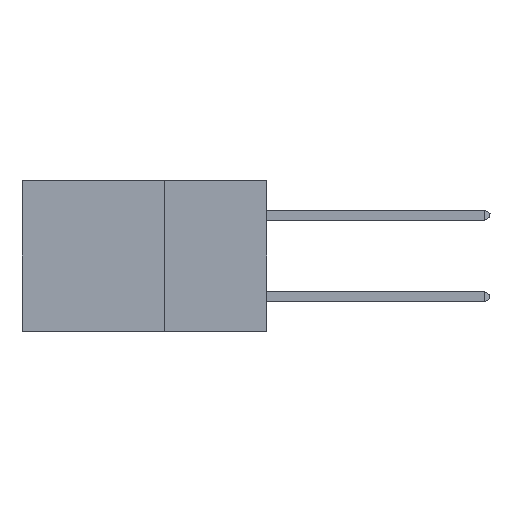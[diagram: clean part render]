
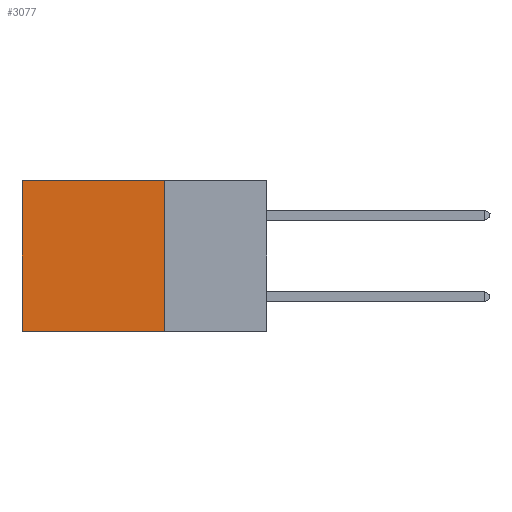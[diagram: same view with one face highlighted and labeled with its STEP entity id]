
A CAD part, left-side view. The second image highlights one B-rep face of the part: STEP entity #3077.
In plain terms, the highlighted planar face has unit normal (-1, 0, 0).
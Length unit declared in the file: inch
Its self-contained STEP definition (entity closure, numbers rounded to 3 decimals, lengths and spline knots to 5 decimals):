
#254 = CARTESIAN_POINT ( 'NONE',  ( 0.2875, 0.25, 0. ) ) ;
#445 = CARTESIAN_POINT ( 'NONE',  ( 0.2875, 0.6, 0. ) ) ;
#1049 = ORIENTED_EDGE ( 'NONE', *, *, #9684, .T. ) ;
#1185 = EDGE_CURVE ( 'NONE', #12153, #7019, #10264, .T. ) ;
#1751 = DIRECTION ( 'NONE',  ( 0., 0., -1. ) ) ;
#2098 = VECTOR ( 'NONE', #1751, 39.37008 ) ;
#2467 = LINE ( 'NONE', #7668, #2098 ) ;
#2470 = CARTESIAN_POINT ( 'NONE',  ( 0.2875, 0.25, -0.37 ) ) ;
#2887 = DIRECTION ( 'NONE',  ( 0., 1., 0. ) ) ;
#2899 = FACE_OUTER_BOUND ( 'NONE', #4478, .T. ) ;
#2956 = CARTESIAN_POINT ( 'NONE',  ( 0.2875, 0.25, 0. ) ) ;
#3077 = ADVANCED_FACE ( 'NONE', ( #2899 ), #14508, .F. ) ;
#3376 = ORIENTED_EDGE ( 'NONE', *, *, #3993, .T. ) ;
#3567 = VERTEX_POINT ( 'NONE', #8154 ) ;
#3993 = EDGE_CURVE ( 'NONE', #12153, #4284, #11089, .T. ) ;
#4284 = VERTEX_POINT ( 'NONE', #445 ) ;
#4478 = EDGE_LOOP ( 'NONE', ( #1049, #7407, #13186, #3376 ) ) ;
#4603 = VECTOR ( 'NONE', #8469, 39.37008 ) ;
#5119 = VECTOR ( 'NONE', #2887, 39.37008 ) ;
#6081 = DIRECTION ( 'NONE',  ( 0., 1., 0. ) ) ;
#7019 = VERTEX_POINT ( 'NONE', #8833 ) ;
#7407 = ORIENTED_EDGE ( 'NONE', *, *, #12311, .F. ) ;
#7668 = CARTESIAN_POINT ( 'NONE',  ( 0.2875, 0.6, 0. ) ) ;
#8104 = LINE ( 'NONE', #2470, #10340 ) ;
#8154 = CARTESIAN_POINT ( 'NONE',  ( 0.2875, 0.6, -0.37 ) ) ;
#8469 = DIRECTION ( 'NONE',  ( 0., 0., -1. ) ) ;
#8833 = CARTESIAN_POINT ( 'NONE',  ( 0.2875, 0.25, -0.37 ) ) ;
#9684 = EDGE_CURVE ( 'NONE', #4284, #3567, #2467, .T. ) ;
#10264 = LINE ( 'NONE', #254, #4603 ) ;
#10340 = VECTOR ( 'NONE', #6081, 39.37008 ) ;
#11084 = AXIS2_PLACEMENT_3D ( 'NONE', #14716, #14483, #14467 ) ;
#11089 = LINE ( 'NONE', #2956, #5119 ) ;
#12153 = VERTEX_POINT ( 'NONE', #12570 ) ;
#12311 = EDGE_CURVE ( 'NONE', #7019, #3567, #8104, .T. ) ;
#12570 = CARTESIAN_POINT ( 'NONE',  ( 0.2875, 0.25, 0. ) ) ;
#13186 = ORIENTED_EDGE ( 'NONE', *, *, #1185, .F. ) ;
#14467 = DIRECTION ( 'NONE',  ( 0., 0., -1. ) ) ;
#14483 = DIRECTION ( 'NONE',  ( 1., 0., 0. ) ) ;
#14508 = PLANE ( 'NONE',  #11084 ) ;
#14716 = CARTESIAN_POINT ( 'NONE',  ( 0.2875, 0.25, 0. ) ) ;
